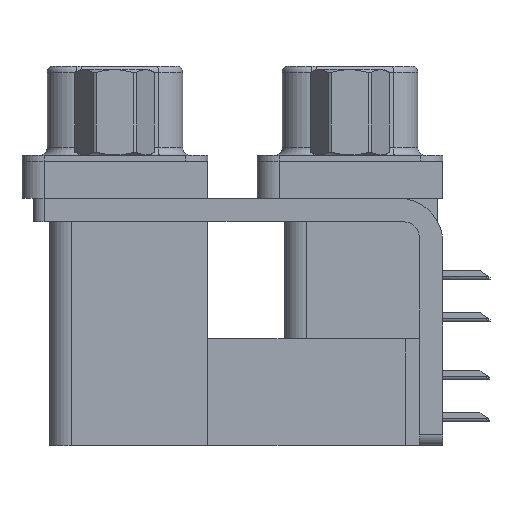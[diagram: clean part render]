
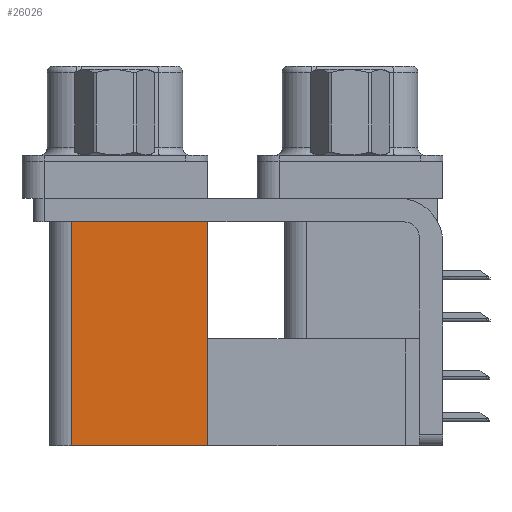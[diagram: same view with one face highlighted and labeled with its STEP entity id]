
A CAD part, left-side view. The second image highlights one B-rep face of the part: STEP entity #26026.
In plain terms, the highlighted planar face has unit normal (-1, 0, 0).
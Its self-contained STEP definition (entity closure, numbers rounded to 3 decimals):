
#140 = DIRECTION ( 'NONE',  ( 0., 1., 0. ) ) ;
#910 = EDGE_CURVE ( 'NONE', #29896, #17261, #19752, .T. ) ;
#1242 = PLANE ( 'NONE',  #34246 ) ;
#1650 = VERTEX_POINT ( 'NONE', #34512 ) ;
#1763 = VECTOR ( 'NONE', #3269, 1000. ) ;
#3269 = DIRECTION ( 'NONE',  ( 0., 0., 1. ) ) ;
#3490 = VECTOR ( 'NONE', #33330, 1000. ) ;
#5526 = CARTESIAN_POINT ( 'NONE',  ( 3.765, 18.8, -19.2 ) ) ;
#8784 = CARTESIAN_POINT ( 'NONE',  ( 3.765, 18.8, -19.2 ) ) ;
#9299 = CARTESIAN_POINT ( 'NONE',  ( 3.765, 18.8, -2.5 ) ) ;
#9755 = ORIENTED_EDGE ( 'NONE', *, *, #17075, .F. ) ;
#10016 = DIRECTION ( 'NONE',  ( 0., 1., 0. ) ) ;
#12299 = VECTOR ( 'NONE', #140, 1000. ) ;
#12590 = DIRECTION ( 'NONE',  ( 0., 0., -1. ) ) ;
#13765 = CARTESIAN_POINT ( 'NONE',  ( 3.765, 9.6, -19.2 ) ) ;
#15861 = CARTESIAN_POINT ( 'NONE',  ( 3.765, 9.6, -2.5 ) ) ;
#16148 = LINE ( 'NONE', #13765, #3490 ) ;
#16460 = EDGE_CURVE ( 'NONE', #1650, #21812, #16148, .T. ) ;
#16789 = VECTOR ( 'NONE', #10016, 1000. ) ;
#17075 = EDGE_CURVE ( 'NONE', #1650, #29896, #25232, .T. ) ;
#17261 = VERTEX_POINT ( 'NONE', #9299 ) ;
#17551 = CARTESIAN_POINT ( 'NONE',  ( 3.765, 9.6, -19.2 ) ) ;
#18384 = ORIENTED_EDGE ( 'NONE', *, *, #16460, .T. ) ;
#19717 = CARTESIAN_POINT ( 'NONE',  ( 3.765, 9.6, -2.5 ) ) ;
#19752 = LINE ( 'NONE', #8784, #1763 ) ;
#21812 = VERTEX_POINT ( 'NONE', #19717 ) ;
#21991 = ORIENTED_EDGE ( 'NONE', *, *, #910, .F. ) ;
#24127 = EDGE_LOOP ( 'NONE', ( #25829, #21991, #9755, #18384 ) ) ;
#25232 = LINE ( 'NONE', #25766, #12299 ) ;
#25766 = CARTESIAN_POINT ( 'NONE',  ( 3.765, 9.6, -19.2 ) ) ;
#25829 = ORIENTED_EDGE ( 'NONE', *, *, #27530, .T. ) ;
#26026 = ADVANCED_FACE ( 'NONE', ( #29056 ), #1242, .F. ) ;
#26320 = DIRECTION ( 'NONE',  ( 1., 0., 0. ) ) ;
#27530 = EDGE_CURVE ( 'NONE', #21812, #17261, #35064, .T. ) ;
#29056 = FACE_OUTER_BOUND ( 'NONE', #24127, .T. ) ;
#29896 = VERTEX_POINT ( 'NONE', #5526 ) ;
#33330 = DIRECTION ( 'NONE',  ( 0., 0., 1. ) ) ;
#34246 = AXIS2_PLACEMENT_3D ( 'NONE', #17551, #26320, #12590 ) ;
#34512 = CARTESIAN_POINT ( 'NONE',  ( 3.765, 9.6, -19.2 ) ) ;
#35064 = LINE ( 'NONE', #15861, #16789 ) ;
